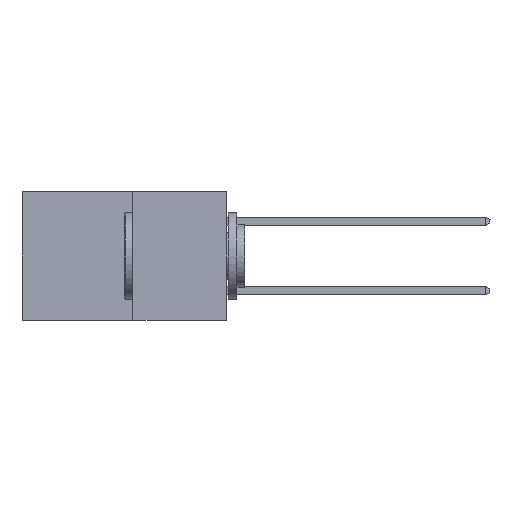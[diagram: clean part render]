
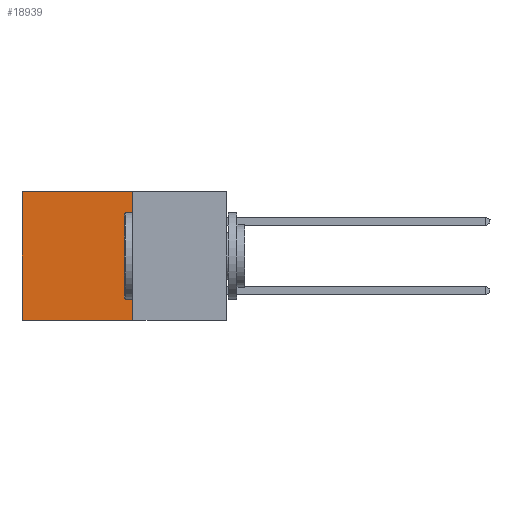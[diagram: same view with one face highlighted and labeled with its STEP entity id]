
A CAD part, left-side view. The second image highlights one B-rep face of the part: STEP entity #18939.
In plain terms, the highlighted planar face has unit normal (-1, 0, 0).
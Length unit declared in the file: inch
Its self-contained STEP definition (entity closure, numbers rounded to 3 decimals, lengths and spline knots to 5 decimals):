
#455 = CARTESIAN_POINT ( 'NONE',  ( 0.277, 0.59, -0.37 ) ) ;
#1878 = ORIENTED_EDGE ( 'NONE', *, *, #2607, .T. ) ;
#2277 = LINE ( 'NONE', #16317, #9588 ) ;
#2607 = EDGE_CURVE ( 'NONE', #14477, #11359, #18892, .T. ) ;
#3194 = ORIENTED_EDGE ( 'NONE', *, *, #7451, .F. ) ;
#4344 = CARTESIAN_POINT ( 'NONE',  ( 0.277, 0.27, 0. ) ) ;
#4797 = EDGE_CURVE ( 'NONE', #4874, #11359, #17842, .T. ) ;
#4874 = VERTEX_POINT ( 'NONE', #8060 ) ;
#5021 = EDGE_LOOP ( 'NONE', ( #1878, #15831, #3194, #14436 ) ) ;
#5281 = VECTOR ( 'NONE', #10244, 39.37008 ) ;
#5355 = VECTOR ( 'NONE', #7811, 39.37008 ) ;
#5432 = PLANE ( 'NONE',  #7408 ) ;
#6513 = VECTOR ( 'NONE', #16143, 39.37008 ) ;
#6966 = CARTESIAN_POINT ( 'NONE',  ( 0.277, 0.59, 0. ) ) ;
#7053 = DIRECTION ( 'NONE',  ( 1., 0., 0. ) ) ;
#7408 = AXIS2_PLACEMENT_3D ( 'NONE', #14863, #7053, #18039 ) ;
#7451 = EDGE_CURVE ( 'NONE', #8493, #4874, #14878, .T. ) ;
#7811 = DIRECTION ( 'NONE',  ( 0., 0., -1. ) ) ;
#8060 = CARTESIAN_POINT ( 'NONE',  ( 0.277, 0.27, -0.37 ) ) ;
#8117 = CARTESIAN_POINT ( 'NONE',  ( 0.277, 0.59, -0.37 ) ) ;
#8493 = VERTEX_POINT ( 'NONE', #4344 ) ;
#9588 = VECTOR ( 'NONE', #17138, 39.37008 ) ;
#10244 = DIRECTION ( 'NONE',  ( 0., 1., 0. ) ) ;
#11359 = VERTEX_POINT ( 'NONE', #455 ) ;
#12780 = EDGE_CURVE ( 'NONE', #8493, #14477, #2277, .T. ) ;
#14436 = ORIENTED_EDGE ( 'NONE', *, *, #12780, .T. ) ;
#14477 = VERTEX_POINT ( 'NONE', #6966 ) ;
#14863 = CARTESIAN_POINT ( 'NONE',  ( 0.277, 0.27, -0.37 ) ) ;
#14878 = LINE ( 'NONE', #19563, #6513 ) ;
#15822 = CARTESIAN_POINT ( 'NONE',  ( 0.277, 0.27, -0.37 ) ) ;
#15831 = ORIENTED_EDGE ( 'NONE', *, *, #4797, .F. ) ;
#16143 = DIRECTION ( 'NONE',  ( 0., 0., -1. ) ) ;
#16317 = CARTESIAN_POINT ( 'NONE',  ( 0.277, 0.27, 0. ) ) ;
#17138 = DIRECTION ( 'NONE',  ( 0., 1., 0. ) ) ;
#17842 = LINE ( 'NONE', #15822, #5281 ) ;
#18039 = DIRECTION ( 'NONE',  ( 0., 0., -1. ) ) ;
#18892 = LINE ( 'NONE', #8117, #5355 ) ;
#18939 = ADVANCED_FACE ( 'NONE', ( #19983 ), #5432, .F. ) ;
#19563 = CARTESIAN_POINT ( 'NONE',  ( 0.277, 0.27, -0.37 ) ) ;
#19983 = FACE_OUTER_BOUND ( 'NONE', #5021, .T. ) ;
